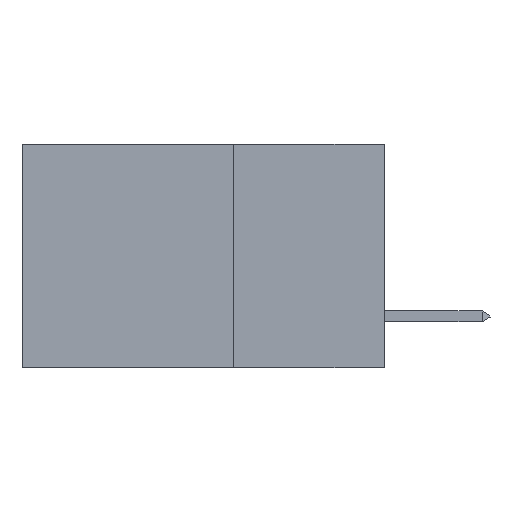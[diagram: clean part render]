
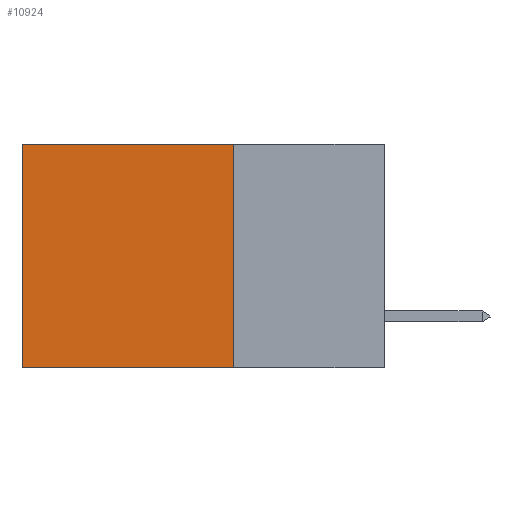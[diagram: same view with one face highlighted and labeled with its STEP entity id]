
A CAD part, left-side view. The second image highlights one B-rep face of the part: STEP entity #10924.
In plain terms, the highlighted planar face has unit normal (-1, 0, 0).
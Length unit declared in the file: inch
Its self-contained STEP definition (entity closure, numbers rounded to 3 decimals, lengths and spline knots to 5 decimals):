
#3458 = FACE_OUTER_BOUND ( 'NONE', #26674, .T. ) ;
#4531 = CARTESIAN_POINT ( 'NONE',  ( 0.2875, 0.25, 0. ) ) ;
#4936 = CARTESIAN_POINT ( 'NONE',  ( 0.2875, 0.25, 0. ) ) ;
#5530 = CARTESIAN_POINT ( 'NONE',  ( 0.2875, 0.6, -0.37 ) ) ;
#6019 = DIRECTION ( 'NONE',  ( 0., 0., -1. ) ) ;
#6353 = EDGE_CURVE ( 'NONE', #24605, #27568, #32392, .T. ) ;
#6753 = VECTOR ( 'NONE', #31921, 39.37008 ) ;
#7383 = DIRECTION ( 'NONE',  ( 0., 1., 0. ) ) ;
#7448 = VERTEX_POINT ( 'NONE', #5530 ) ;
#10924 = ADVANCED_FACE ( 'NONE', ( #3458 ), #16577, .F. ) ;
#12871 = AXIS2_PLACEMENT_3D ( 'NONE', #13925, #29047, #6019 ) ;
#12961 = ORIENTED_EDGE ( 'NONE', *, *, #30573, .F. ) ;
#13730 = CARTESIAN_POINT ( 'NONE',  ( 0.2875, 0.25, -0.37 ) ) ;
#13903 = LINE ( 'NONE', #21528, #6753 ) ;
#13925 = CARTESIAN_POINT ( 'NONE',  ( 0.2875, 0.25, 0. ) ) ;
#16577 = PLANE ( 'NONE',  #12871 ) ;
#17342 = CARTESIAN_POINT ( 'NONE',  ( 0.2875, 0.25, 0. ) ) ;
#17638 = VECTOR ( 'NONE', #7383, 39.37008 ) ;
#18990 = ORIENTED_EDGE ( 'NONE', *, *, #31790, .F. ) ;
#20088 = DIRECTION ( 'NONE',  ( 0., 0., -1. ) ) ;
#20198 = DIRECTION ( 'NONE',  ( 0., 1., 0. ) ) ;
#20479 = LINE ( 'NONE', #17342, #26870 ) ;
#21528 = CARTESIAN_POINT ( 'NONE',  ( 0.2875, 0.6, 0. ) ) ;
#24007 = CARTESIAN_POINT ( 'NONE',  ( 0.2875, 0.6, 0. ) ) ;
#24605 = VERTEX_POINT ( 'NONE', #4531 ) ;
#25875 = ORIENTED_EDGE ( 'NONE', *, *, #6353, .T. ) ;
#25881 = VERTEX_POINT ( 'NONE', #13730 ) ;
#26674 = EDGE_LOOP ( 'NONE', ( #29931, #12961, #18990, #25875 ) ) ;
#26870 = VECTOR ( 'NONE', #20088, 39.37008 ) ;
#27568 = VERTEX_POINT ( 'NONE', #24007 ) ;
#29047 = DIRECTION ( 'NONE',  ( 1., 0., 0. ) ) ;
#29054 = EDGE_CURVE ( 'NONE', #27568, #7448, #13903, .T. ) ;
#29315 = LINE ( 'NONE', #30574, #29672 ) ;
#29672 = VECTOR ( 'NONE', #20198, 39.37008 ) ;
#29931 = ORIENTED_EDGE ( 'NONE', *, *, #29054, .T. ) ;
#30573 = EDGE_CURVE ( 'NONE', #25881, #7448, #29315, .T. ) ;
#30574 = CARTESIAN_POINT ( 'NONE',  ( 0.2875, 0.25, -0.37 ) ) ;
#31790 = EDGE_CURVE ( 'NONE', #24605, #25881, #20479, .T. ) ;
#31921 = DIRECTION ( 'NONE',  ( 0., 0., -1. ) ) ;
#32392 = LINE ( 'NONE', #4936, #17638 ) ;
